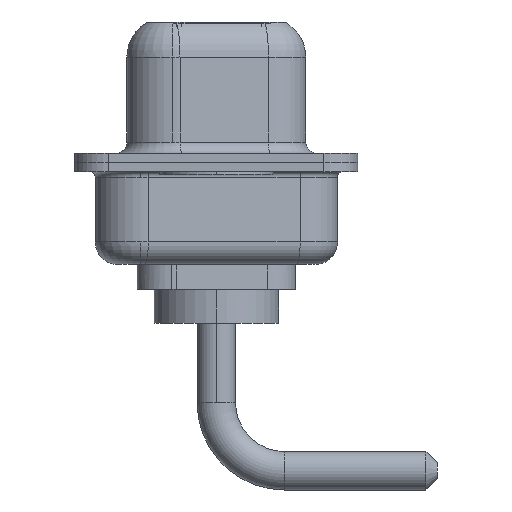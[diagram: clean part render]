
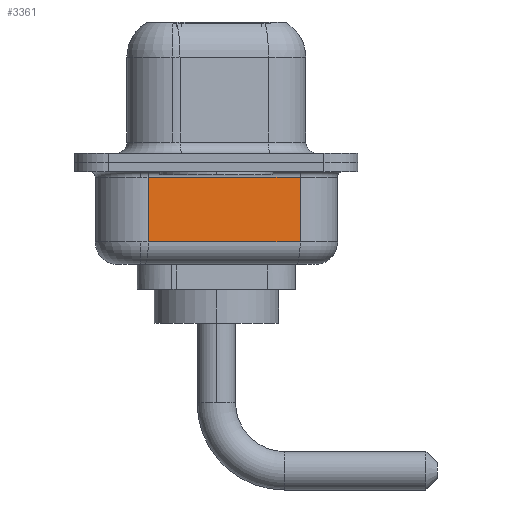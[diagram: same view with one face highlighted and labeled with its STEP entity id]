
A CAD part, left-side view. The second image highlights one B-rep face of the part: STEP entity #3361.
In plain terms, the highlighted planar face has unit normal (-0.985, -0.174, 0).
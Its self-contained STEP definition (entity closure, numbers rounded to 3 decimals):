
#61 = VERTEX_POINT ( 'NONE', #2522 ) ;
#100 = CARTESIAN_POINT ( 'NONE',  ( 2.855, 3.003, -3.5 ) ) ;
#507 = VERTEX_POINT ( 'NONE', #10243 ) ;
#830 = CARTESIAN_POINT ( 'NONE',  ( 4.037, -3.697, -0.65 ) ) ;
#834 = VECTOR ( 'NONE', #8544, 1000. ) ;
#1285 = EDGE_CURVE ( 'NONE', #2729, #61, #5099, .T. ) ;
#1876 = CARTESIAN_POINT ( 'NONE',  ( 2.855, 3.003, -3.5 ) ) ;
#2522 = CARTESIAN_POINT ( 'NONE',  ( 4.037, -3.697, -3.5 ) ) ;
#2563 = DIRECTION ( 'NONE',  ( -0.174, 0.985, 0. ) ) ;
#2663 = LINE ( 'NONE', #9402, #4426 ) ;
#2729 = VERTEX_POINT ( 'NONE', #1876 ) ;
#3361 = ADVANCED_FACE ( 'NONE', ( #9292 ), #6969, .F. ) ;
#3423 = EDGE_CURVE ( 'NONE', #61, #9679, #2663, .T. ) ;
#3627 = EDGE_LOOP ( 'NONE', ( #4452, #5366, #9550, #5998 ) ) ;
#3707 = LINE ( 'NONE', #7082, #8051 ) ;
#4361 = DIRECTION ( 'NONE',  ( -0.174, 0.985, 0. ) ) ;
#4426 = VECTOR ( 'NONE', #6023, 1000. ) ;
#4452 = ORIENTED_EDGE ( 'NONE', *, *, #6415, .F. ) ;
#5099 = LINE ( 'NONE', #100, #834 ) ;
#5366 = ORIENTED_EDGE ( 'NONE', *, *, #1285, .T. ) ;
#5369 = DIRECTION ( 'NONE',  ( 0., 0., 1. ) ) ;
#5998 = ORIENTED_EDGE ( 'NONE', *, *, #8782, .T. ) ;
#6023 = DIRECTION ( 'NONE',  ( 0., 0., 1. ) ) ;
#6089 = CARTESIAN_POINT ( 'NONE',  ( 2.855, 3.003, -4.5 ) ) ;
#6415 = EDGE_CURVE ( 'NONE', #2729, #507, #3707, .T. ) ;
#6852 = CARTESIAN_POINT ( 'NONE',  ( 2.855, 3.003, -0.65 ) ) ;
#6969 = PLANE ( 'NONE',  #10466 ) ;
#7082 = CARTESIAN_POINT ( 'NONE',  ( 2.855, 3.003, -4.5 ) ) ;
#8051 = VECTOR ( 'NONE', #5369, 1000. ) ;
#8544 = DIRECTION ( 'NONE',  ( 0.174, -0.985, 0. ) ) ;
#8627 = DIRECTION ( 'NONE',  ( 0.985, 0.174, 0. ) ) ;
#8738 = VECTOR ( 'NONE', #4361, 1000. ) ;
#8782 = EDGE_CURVE ( 'NONE', #9679, #507, #9885, .T. ) ;
#9292 = FACE_OUTER_BOUND ( 'NONE', #3627, .T. ) ;
#9402 = CARTESIAN_POINT ( 'NONE',  ( 4.037, -3.697, -4.5 ) ) ;
#9550 = ORIENTED_EDGE ( 'NONE', *, *, #3423, .T. ) ;
#9679 = VERTEX_POINT ( 'NONE', #830 ) ;
#9885 = LINE ( 'NONE', #6852, #8738 ) ;
#10243 = CARTESIAN_POINT ( 'NONE',  ( 2.855, 3.003, -0.65 ) ) ;
#10466 = AXIS2_PLACEMENT_3D ( 'NONE', #6089, #8627, #2563 ) ;
